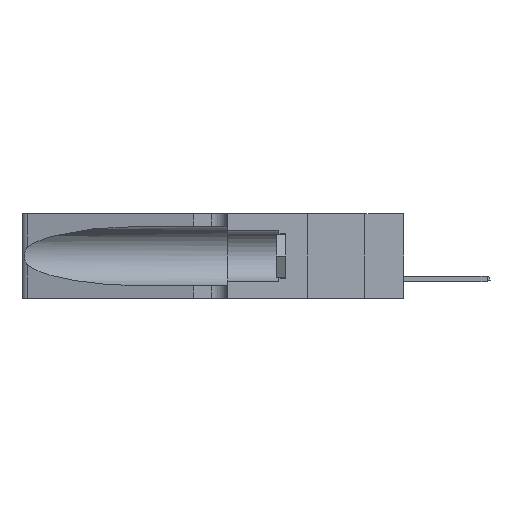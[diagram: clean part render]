
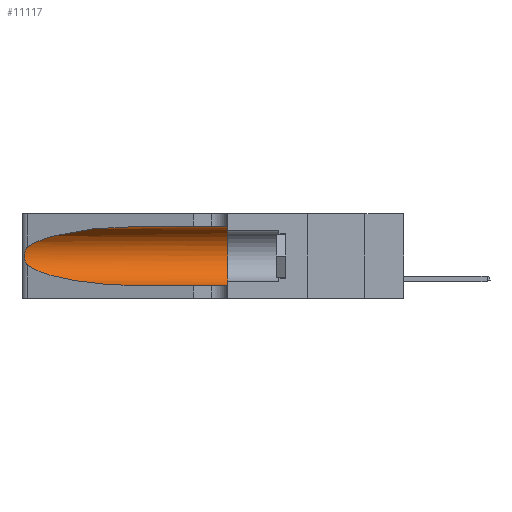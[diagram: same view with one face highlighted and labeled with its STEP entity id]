
A CAD part, left-side view. The second image highlights one B-rep face of the part: STEP entity #11117.
In plain terms, the highlighted cylindrical face has radius 3.308 mm (diameter 6.617 mm), a partial arc.
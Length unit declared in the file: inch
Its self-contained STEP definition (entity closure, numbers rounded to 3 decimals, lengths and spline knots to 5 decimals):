
#403 = CARTESIAN_POINT ( 'NONE',  ( 0.1305, 0.35, 0.31525 ) ) ;
#883 = CARTESIAN_POINT ( 'NONE',  ( 0.25487, 1.22718, 0.22369 ) ) ;
#961 = CARTESIAN_POINT ( 'NONE',  ( 0.2373, 1.15595, 0.08982 ) ) ;
#1106 = ORIENTED_EDGE ( 'NONE', *, *, #15177, .T. ) ;
#1129 = CARTESIAN_POINT ( 'NONE',  ( 0.25487, 1.22718, 0.14631 ) ) ;
#2293 = VERTEX_POINT ( 'NONE', #403 ) ;
#2457 = VERTEX_POINT ( 'NONE', #16744 ) ;
#2748 = VERTEX_POINT ( 'NONE', #21879 ) ;
#3152 = CARTESIAN_POINT ( 'NONE',  ( 0.26017, 1.23833, 0.17102 ) ) ;
#3553 = CARTESIAN_POINT ( 'NONE',  ( 0.25555, 1.22994, 0.2215 ) ) ;
#3631 = ORIENTED_EDGE ( 'NONE', *, *, #11087, .T. ) ;
#3836 = DIRECTION ( 'NONE',  ( 0., -1., 0. ) ) ;
#3890 = CARTESIAN_POINT ( 'NONE',  ( 0.18966, 0.96281, 0.31525 ) ) ;
#4379 = AXIS2_PLACEMENT_3D ( 'NONE', #4648, #10370, #11072 ) ;
#4648 = CARTESIAN_POINT ( 'NONE',  ( 0.1305, 1.61858, 0.185 ) ) ;
#4697 = CARTESIAN_POINT ( 'NONE',  ( 0.18966, 0.96281, 0.05475 ) ) ;
#4852 = CARTESIAN_POINT ( 'NONE',  ( 0.25487, 1.22718, 0.22369 ) ) ;
#4940 = CARTESIAN_POINT ( 'NONE',  ( 0.25555, 1.22993, 0.14849 ) ) ;
#4956 = CARTESIAN_POINT ( 'NONE',  ( 0.26018, 1.23835, 0.19895 ) ) ;
#5519 = EDGE_CURVE ( 'NONE', #2293, #2748, #8175, .T. ) ;
#6107 = CARTESIAN_POINT ( 'NONE',  ( 0.25487, 1.22718, 0.22369 ) ) ;
#6677 = LINE ( 'NONE', #21425, #13408 ) ;
#6882 = CARTESIAN_POINT ( 'NONE',  ( 0.25487, 1.22718, 0.14631 ) ) ;
#6898 = CARTESIAN_POINT ( 'NONE',  ( 0.26075, 1.23896, 0.19203 ) ) ;
#7220 = VERTEX_POINT ( 'NONE', #21382 ) ;
#8175 = CIRCLE ( 'NONE', #20031, 0.13025 ) ;
#8474 = CARTESIAN_POINT ( 'NONE',  ( 0.1305, 0.72297, 0.05475 ) ) ;
#8916 = CARTESIAN_POINT ( 'NONE',  ( 0.1305, 1.61858, 0.05475 ) ) ;
#9086 = EDGE_CURVE ( 'NONE', #7220, #23894, #18519, .T. ) ;
#9130 = ORIENTED_EDGE ( 'NONE', *, *, #23506, .T. ) ;
#10034 = CARTESIAN_POINT ( 'NONE',  ( 0.1305, 0.72297, 0.31525 ) ) ;
#10370 = DIRECTION ( 'NONE',  ( 0., -1., 0. ) ) ;
#10498 = DIRECTION ( 'NONE',  ( 0., 1., 0. ) ) ;
#10753 = CYLINDRICAL_SURFACE ( 'NONE', #4379, 0.13025 ) ;
#11072 = DIRECTION ( 'NONE',  ( 0., 0., -1. ) ) ;
#11087 = EDGE_CURVE ( 'NONE', #23894, #2457, #23047, .T. ) ;
#11117 = ADVANCED_FACE ( 'NONE', ( #15930 ), #10753, .F. ) ;
#12520 = DIRECTION ( 'NONE',  ( 0., 0., 1. ) ) ;
#13028 = LINE ( 'NONE', #8916, #13649 ) ;
#13408 = VECTOR ( 'NONE', #3836, 39.37008 ) ;
#13649 = VECTOR ( 'NONE', #18798, 39.37008 ) ;
#14621 =( BOUNDED_CURVE ( )  B_SPLINE_CURVE ( 3, ( #1129, #961, #4697, #22281 ),
 .UNSPECIFIED., .F., .T. ) 
 B_SPLINE_CURVE_WITH_KNOTS ( ( 4, 4 ),
 ( 3.44316, 4.71239 ),
 .UNSPECIFIED. ) 
 CURVE ( )  GEOMETRIC_REPRESENTATION_ITEM ( )  RATIONAL_B_SPLINE_CURVE ( ( 1., 0.87, 0.87, 1. ) ) 
 REPRESENTATION_ITEM ( '' )  );
#14769 = CARTESIAN_POINT ( 'NONE',  ( 0.25854, 1.2359, 0.20912 ) ) ;
#15177 = EDGE_CURVE ( 'NONE', #2457, #15999, #14621, .T. ) ;
#15930 = FACE_OUTER_BOUND ( 'NONE', #22352, .T. ) ;
#15999 = VERTEX_POINT ( 'NONE', #8474 ) ;
#16744 = CARTESIAN_POINT ( 'NONE',  ( 0.25487, 1.22718, 0.14631 ) ) ;
#16975 = ORIENTED_EDGE ( 'NONE', *, *, #5519, .F. ) ;
#18074 = ORIENTED_EDGE ( 'NONE', *, *, #9086, .T. ) ;
#18337 = CARTESIAN_POINT ( 'NONE',  ( 0.1305, 0.35, 0.185 ) ) ;
#18519 =( BOUNDED_CURVE ( )  B_SPLINE_CURVE ( 3, ( #10034, #3890, #19517, #6107 ),
 .UNSPECIFIED., .F., .T. ) 
 B_SPLINE_CURVE_WITH_KNOTS ( ( 4, 4 ),
 ( 1.5708, 2.84003 ),
 .UNSPECIFIED. ) 
 CURVE ( )  GEOMETRIC_REPRESENTATION_ITEM ( )  RATIONAL_B_SPLINE_CURVE ( ( 1., 0.87, 0.87, 1. ) ) 
 REPRESENTATION_ITEM ( '' )  );
#18591 = CARTESIAN_POINT ( 'NONE',  ( 0.25639, 1.23186, 0.15144 ) ) ;
#18642 = CARTESIAN_POINT ( 'NONE',  ( 0.25639, 1.23184, 0.21858 ) ) ;
#18697 = CARTESIAN_POINT ( 'NONE',  ( 0.25856, 1.23593, 0.16098 ) ) ;
#18798 = DIRECTION ( 'NONE',  ( 0., -1., 0. ) ) ;
#19517 = CARTESIAN_POINT ( 'NONE',  ( 0.2373, 1.15595, 0.28018 ) ) ;
#19615 = EDGE_CURVE ( 'NONE', #7220, #2293, #6677, .T. ) ;
#19692 = ORIENTED_EDGE ( 'NONE', *, *, #19615, .F. ) ;
#20031 = AXIS2_PLACEMENT_3D ( 'NONE', #18337, #10498, #12520 ) ;
#21382 = CARTESIAN_POINT ( 'NONE',  ( 0.1305, 0.72297, 0.31525 ) ) ;
#21425 = CARTESIAN_POINT ( 'NONE',  ( 0.1305, 1.61858, 0.31525 ) ) ;
#21879 = CARTESIAN_POINT ( 'NONE',  ( 0.1305, 0.35, 0.05475 ) ) ;
#22281 = CARTESIAN_POINT ( 'NONE',  ( 0.1305, 0.72297, 0.05475 ) ) ;
#22352 = EDGE_LOOP ( 'NONE', ( #18074, #3631, #1106, #9130, #16975, #19692 ) ) ;
#22536 = CARTESIAN_POINT ( 'NONE',  ( 0.26075, 1.23896, 0.178 ) ) ;
#22871 = CARTESIAN_POINT ( 'NONE',  ( 0.25789, 1.23486, 0.15765 ) ) ;
#23047 = B_SPLINE_CURVE_WITH_KNOTS ( 'NONE', 3,
 ( #4852, #3553, #18642, #23399, #14769, #4956, #6898, #22536, #3152, #18697, #22871, #18591, #4940, #6882 ),
 .UNSPECIFIED., .F., .F.,
 ( 4, 2, 2, 2, 2, 2, 4 ),
 ( 0., 0.00027, 0.00053, 0.00107, 0.0016, 0.00187, 0.00214 ),
 .UNSPECIFIED. ) ;
#23399 = CARTESIAN_POINT ( 'NONE',  ( 0.25787, 1.23484, 0.2124 ) ) ;
#23506 = EDGE_CURVE ( 'NONE', #15999, #2748, #13028, .T. ) ;
#23894 = VERTEX_POINT ( 'NONE', #883 ) ;
